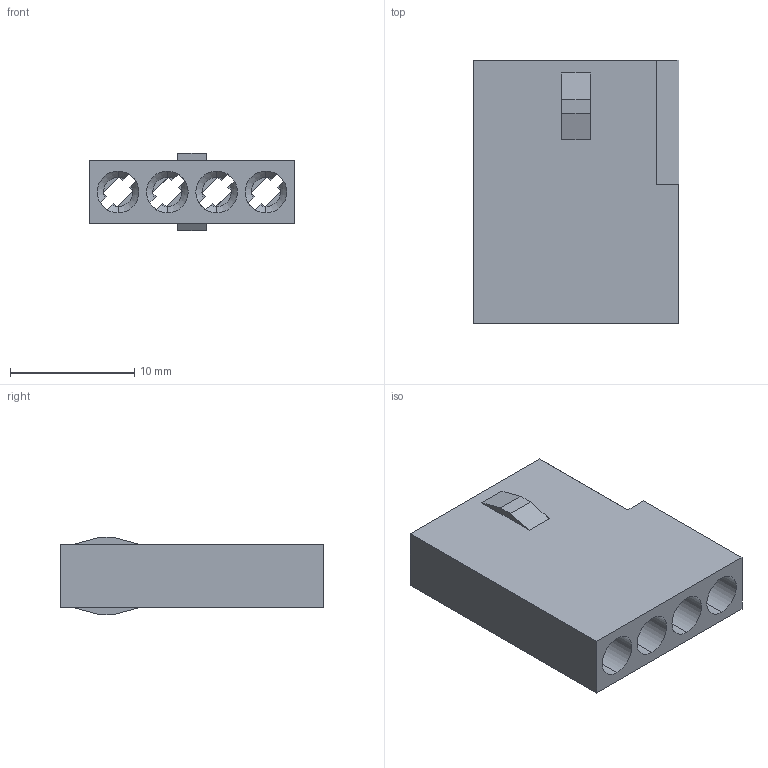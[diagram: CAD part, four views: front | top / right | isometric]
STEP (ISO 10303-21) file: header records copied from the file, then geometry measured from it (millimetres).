
FILE_DESCRIPTION (( 'STEP AP203' ), '1' );
FILE_NAME ('556-004-000-101.STEP', '2020-03-13T14:29:13', ( '' ), ( '' ), 'SwSTEP 2.0', 'SolidWorks 2016', '' );
FILE_SCHEMA (( 'CONFIG_CONTROL_DESIGN' ));
Length unit declared in the file: millimetre
Products named in the file (2): 556-004-000-101; 556-210-001_556-004-000-101
Assembly tree (1 placements, depth 2):
  556-004-000-101
    556-210-001_556-004-000-101
Bounding box: 16.54 x 21.21 x 6.22 mm (x, y, z)
Volume: 1144.5 mm3; surface area: 1998.5 mm2
Topology: 1 solids, 1 shells, 124 faces, 352 edges, 232 vertices
Faces by surface type: plane 92, cylinder 24, cone 8
Entity records: 4272 total; most frequent: CARTESIAN_POINT 856, ORIENTED_EDGE 704, DIRECTION 640, EDGE_CURVE 352, VERTEX_POINT 232, VECTOR 224, LINE 224, AXIS2_PLACEMENT_3D 208
